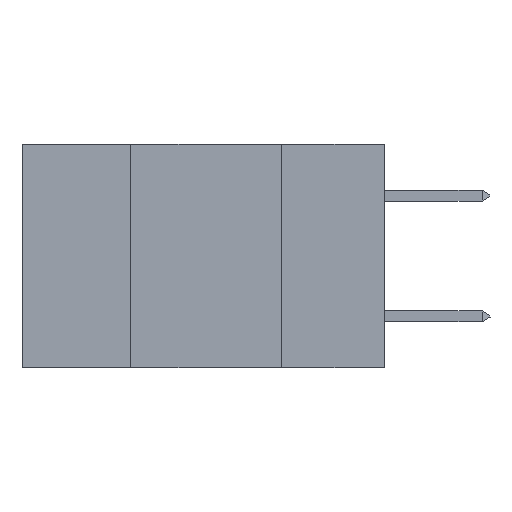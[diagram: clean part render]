
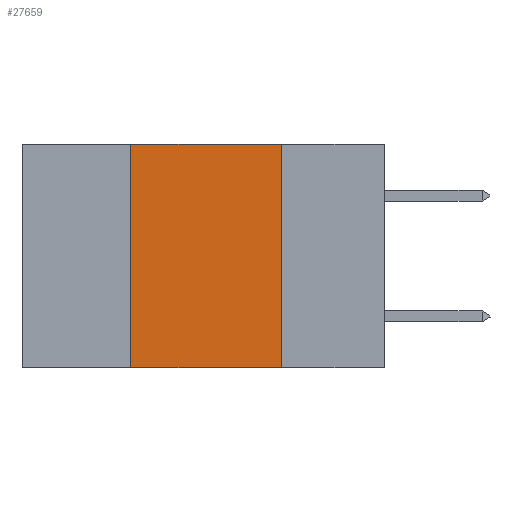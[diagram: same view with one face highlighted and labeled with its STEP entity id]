
A CAD part, left-side view. The second image highlights one B-rep face of the part: STEP entity #27659.
In plain terms, the highlighted planar face has unit normal (-1, 0, 0).
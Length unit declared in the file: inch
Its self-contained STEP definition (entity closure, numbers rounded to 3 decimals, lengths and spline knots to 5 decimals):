
#1340 = AXIS2_PLACEMENT_3D ( 'NONE', #4824, #1735, #7760 ) ;
#1735 = DIRECTION ( 'NONE',  ( 1., 0., 0. ) ) ;
#1886 = EDGE_LOOP ( 'NONE', ( #32886, #38124, #2245, #14725 ) ) ;
#2207 = CARTESIAN_POINT ( 'NONE',  ( 0., 0.42, 0. ) ) ;
#2245 = ORIENTED_EDGE ( 'NONE', *, *, #37942, .F. ) ;
#3081 = LINE ( 'NONE', #26664, #7380 ) ;
#4824 = CARTESIAN_POINT ( 'NONE',  ( 0., 0.6, 0. ) ) ;
#5201 = DIRECTION ( 'NONE',  ( 0., -1., 0. ) ) ;
#5911 = LINE ( 'NONE', #22604, #6361 ) ;
#6361 = VECTOR ( 'NONE', #13934, 39.37008 ) ;
#7176 = VECTOR ( 'NONE', #24042, 39.37008 ) ;
#7380 = VECTOR ( 'NONE', #5201, 39.37008 ) ;
#7760 = DIRECTION ( 'NONE',  ( 0., 0., -1. ) ) ;
#8469 = VERTEX_POINT ( 'NONE', #12035 ) ;
#10638 = VERTEX_POINT ( 'NONE', #16982 ) ;
#12035 = CARTESIAN_POINT ( 'NONE',  ( 0., 0.17, 0. ) ) ;
#13934 = DIRECTION ( 'NONE',  ( 0., 0., -1. ) ) ;
#14725 = ORIENTED_EDGE ( 'NONE', *, *, #20803, .T. ) ;
#16982 = CARTESIAN_POINT ( 'NONE',  ( 0., 0.42, -0.37 ) ) ;
#18255 = LINE ( 'NONE', #24310, #7176 ) ;
#20803 = EDGE_CURVE ( 'NONE', #10638, #37215, #3081, .T. ) ;
#21313 = EDGE_CURVE ( 'NONE', #8469, #37215, #5911, .T. ) ;
#21758 = CARTESIAN_POINT ( 'NONE',  ( 0., 0.17, -0.37 ) ) ;
#22098 = DIRECTION ( 'NONE',  ( 0., 0., 1. ) ) ;
#22604 = CARTESIAN_POINT ( 'NONE',  ( 0., 0.17, 0. ) ) ;
#23610 = VERTEX_POINT ( 'NONE', #2207 ) ;
#24042 = DIRECTION ( 'NONE',  ( 0., -1., 0. ) ) ;
#24310 = CARTESIAN_POINT ( 'NONE',  ( 0., 0.6, 0. ) ) ;
#25192 = VECTOR ( 'NONE', #22098, 39.37008 ) ;
#26664 = CARTESIAN_POINT ( 'NONE',  ( 0., 0.6, -0.37 ) ) ;
#27659 = ADVANCED_FACE ( 'NONE', ( #32809 ), #35254, .F. ) ;
#28269 = CARTESIAN_POINT ( 'NONE',  ( 0., 0.42, 0. ) ) ;
#32809 = FACE_OUTER_BOUND ( 'NONE', #1886, .T. ) ;
#32886 = ORIENTED_EDGE ( 'NONE', *, *, #21313, .F. ) ;
#33330 = LINE ( 'NONE', #28269, #25192 ) ;
#35254 = PLANE ( 'NONE',  #1340 ) ;
#37215 = VERTEX_POINT ( 'NONE', #21758 ) ;
#37942 = EDGE_CURVE ( 'NONE', #10638, #23610, #33330, .T. ) ;
#38124 = ORIENTED_EDGE ( 'NONE', *, *, #38814, .F. ) ;
#38814 = EDGE_CURVE ( 'NONE', #23610, #8469, #18255, .T. ) ;
